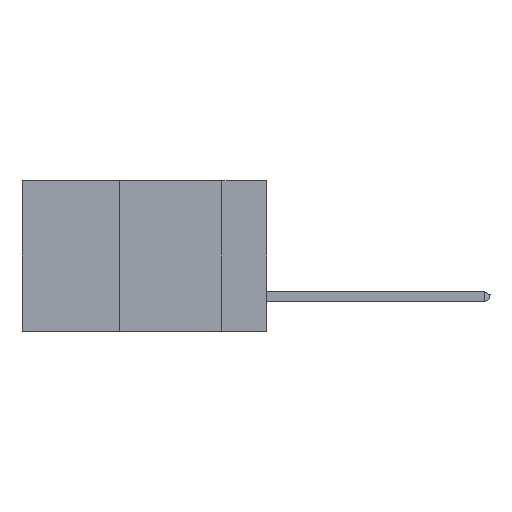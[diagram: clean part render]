
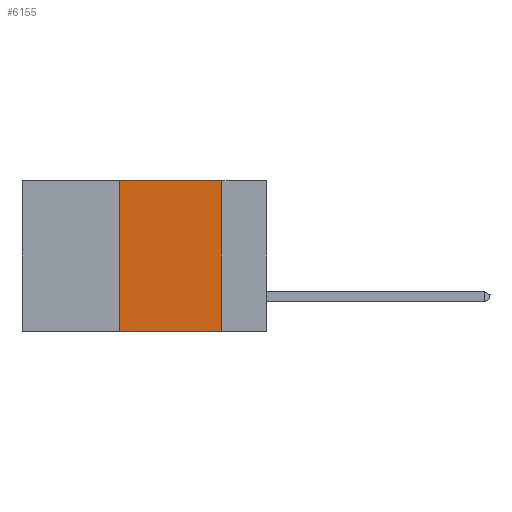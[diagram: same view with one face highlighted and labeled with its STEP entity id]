
A CAD part, left-side view. The second image highlights one B-rep face of the part: STEP entity #6155.
In plain terms, the highlighted planar face has unit normal (-1, 0, 0).
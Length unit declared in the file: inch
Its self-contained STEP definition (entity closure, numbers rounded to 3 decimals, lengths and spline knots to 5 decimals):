
#75 = VERTEX_POINT ( 'NONE', #15484 ) ;
#348 = EDGE_CURVE ( 'NONE', #11555, #16099, #11246, .T. ) ;
#352 = ORIENTED_EDGE ( 'NONE', *, *, #348, .T. ) ;
#492 = VERTEX_POINT ( 'NONE', #9021 ) ;
#4083 = EDGE_CURVE ( 'NONE', #75, #16099, #8587, .T. ) ;
#5197 = LINE ( 'NONE', #10441, #5282 ) ;
#5282 = VECTOR ( 'NONE', #11164, 39.37008 ) ;
#5572 = PLANE ( 'NONE',  #10673 ) ;
#6155 = ADVANCED_FACE ( 'NONE', ( #7112 ), #5572, .F. ) ;
#6242 = DIRECTION ( 'NONE',  ( 0., -1., 0. ) ) ;
#6299 = EDGE_CURVE ( 'NONE', #492, #75, #5197, .T. ) ;
#6339 = LINE ( 'NONE', #16599, #12093 ) ;
#6493 = VECTOR ( 'NONE', #6242, 39.37008 ) ;
#6675 = CARTESIAN_POINT ( 'NONE',  ( 0., 0.36, -0.37 ) ) ;
#7112 = FACE_OUTER_BOUND ( 'NONE', #12867, .T. ) ;
#8077 = VECTOR ( 'NONE', #9845, 39.37008 ) ;
#8587 = LINE ( 'NONE', #11140, #8077 ) ;
#8803 = ORIENTED_EDGE ( 'NONE', *, *, #4083, .F. ) ;
#8880 = ORIENTED_EDGE ( 'NONE', *, *, #6299, .F. ) ;
#9021 = CARTESIAN_POINT ( 'NONE',  ( 0., 0.36, 0. ) ) ;
#9547 = DIRECTION ( 'NONE',  ( 1., 0., 0. ) ) ;
#9845 = DIRECTION ( 'NONE',  ( 0., 0., -1. ) ) ;
#10441 = CARTESIAN_POINT ( 'NONE',  ( 0., 0.6, 0. ) ) ;
#10673 = AXIS2_PLACEMENT_3D ( 'NONE', #15916, #9547, #12259 ) ;
#11140 = CARTESIAN_POINT ( 'NONE',  ( 0., 0.11, 0. ) ) ;
#11164 = DIRECTION ( 'NONE',  ( 0., -1., 0. ) ) ;
#11246 = LINE ( 'NONE', #14981, #6493 ) ;
#11268 = DIRECTION ( 'NONE',  ( 0., 0., 1. ) ) ;
#11395 = CARTESIAN_POINT ( 'NONE',  ( 0., 0.11, -0.37 ) ) ;
#11555 = VERTEX_POINT ( 'NONE', #6675 ) ;
#12093 = VECTOR ( 'NONE', #11268, 39.37008 ) ;
#12259 = DIRECTION ( 'NONE',  ( 0., 0., -1. ) ) ;
#12867 = EDGE_LOOP ( 'NONE', ( #8803, #8880, #13577, #352 ) ) ;
#13577 = ORIENTED_EDGE ( 'NONE', *, *, #14003, .F. ) ;
#14003 = EDGE_CURVE ( 'NONE', #11555, #492, #6339, .T. ) ;
#14981 = CARTESIAN_POINT ( 'NONE',  ( 0., 0.6, -0.37 ) ) ;
#15484 = CARTESIAN_POINT ( 'NONE',  ( 0., 0.11, 0. ) ) ;
#15916 = CARTESIAN_POINT ( 'NONE',  ( 0., 0.6, 0. ) ) ;
#16099 = VERTEX_POINT ( 'NONE', #11395 ) ;
#16599 = CARTESIAN_POINT ( 'NONE',  ( 0., 0.36, 0. ) ) ;
